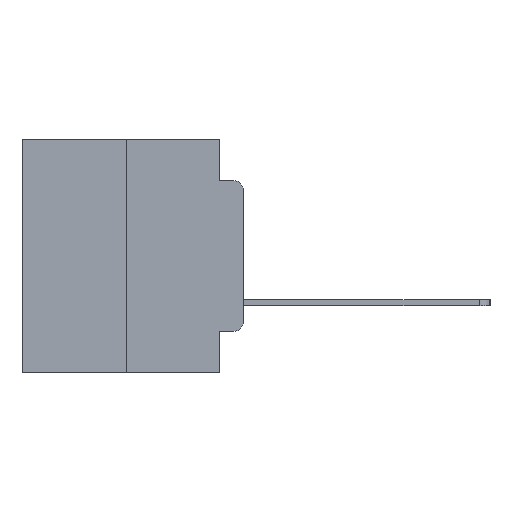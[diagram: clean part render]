
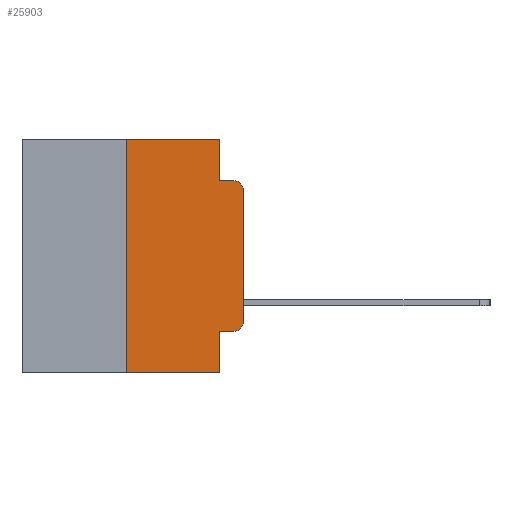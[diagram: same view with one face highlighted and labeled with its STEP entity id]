
A CAD part, left-side view. The second image highlights one B-rep face of the part: STEP entity #25903.
In plain terms, the highlighted planar face has unit normal (-1, 0, 0).
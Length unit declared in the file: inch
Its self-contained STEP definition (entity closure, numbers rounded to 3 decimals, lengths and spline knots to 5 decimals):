
#150 = CARTESIAN_POINT ( 'NONE',  ( 0., 0., -0.1085 ) ) ;
#372 = CARTESIAN_POINT ( 'NONE',  ( 0., 0.473, 0. ) ) ;
#815 = DIRECTION ( 'NONE',  ( 0., 0., 1. ) ) ;
#927 = DIRECTION ( 'NONE',  ( 0., 0., -1. ) ) ;
#1310 = CARTESIAN_POINT ( 'NONE',  ( 0., 0.02, -0.4115 ) ) ;
#1824 = CARTESIAN_POINT ( 'NONE',  ( 0., 0.02, -0.0885 ) ) ;
#1943 = CARTESIAN_POINT ( 'NONE',  ( 0., 0.051, 0. ) ) ;
#2210 = CIRCLE ( 'NONE', #12463, 0.02 ) ;
#2427 = CARTESIAN_POINT ( 'NONE',  ( 0., 0., 0. ) ) ;
#3663 = ORIENTED_EDGE ( 'NONE', *, *, #15110, .T. ) ;
#3817 = EDGE_CURVE ( 'NONE', #10203, #20519, #4267, .T. ) ;
#3851 = EDGE_CURVE ( 'NONE', #9845, #5851, #14530, .T. ) ;
#3986 = VECTOR ( 'NONE', #6783, 39.37008 ) ;
#4055 = DIRECTION ( 'NONE',  ( 0., 0., -1. ) ) ;
#4267 = CIRCLE ( 'NONE', #9182, 0.02 ) ;
#4334 = VECTOR ( 'NONE', #20975, 39.37008 ) ;
#4427 = CARTESIAN_POINT ( 'NONE',  ( 0., 0.051, 0. ) ) ;
#5043 = LINE ( 'NONE', #1943, #15949 ) ;
#5316 = CARTESIAN_POINT ( 'NONE',  ( 0., 0.25, -0.5 ) ) ;
#5504 = EDGE_CURVE ( 'NONE', #13456, #21660, #2210, .T. ) ;
#5851 = VERTEX_POINT ( 'NONE', #18523 ) ;
#6529 = CARTESIAN_POINT ( 'NONE',  ( 0., 0.051, -0.0885 ) ) ;
#6564 = EDGE_CURVE ( 'NONE', #21660, #10203, #19467, .T. ) ;
#6783 = DIRECTION ( 'NONE',  ( 0., -1., 0. ) ) ;
#7154 = VERTEX_POINT ( 'NONE', #18896 ) ;
#7891 = ORIENTED_EDGE ( 'NONE', *, *, #22722, .F. ) ;
#8489 = VECTOR ( 'NONE', #26136, 39.37008 ) ;
#8744 = ORIENTED_EDGE ( 'NONE', *, *, #20754, .F. ) ;
#9182 = AXIS2_PLACEMENT_3D ( 'NONE', #19022, #16588, #16552 ) ;
#9845 = VERTEX_POINT ( 'NONE', #5316 ) ;
#10203 = VERTEX_POINT ( 'NONE', #150 ) ;
#10524 = DIRECTION ( 'NONE',  ( 0., 0., -1. ) ) ;
#10583 = AXIS2_PLACEMENT_3D ( 'NONE', #372, #25048, #12928 ) ;
#11063 = LINE ( 'NONE', #11196, #17168 ) ;
#11196 = CARTESIAN_POINT ( 'NONE',  ( 0., 0.25, 0. ) ) ;
#12216 = ORIENTED_EDGE ( 'NONE', *, *, #3851, .T. ) ;
#12463 = AXIS2_PLACEMENT_3D ( 'NONE', #25460, #13337, #927 ) ;
#12928 = DIRECTION ( 'NONE',  ( 0., 0., -1. ) ) ;
#13304 = CARTESIAN_POINT ( 'NONE',  ( 0., 0.473, 0. ) ) ;
#13337 = DIRECTION ( 'NONE',  ( -1., 0., 0. ) ) ;
#13456 = VERTEX_POINT ( 'NONE', #1310 ) ;
#14033 = VECTOR ( 'NONE', #18833, 39.37008 ) ;
#14147 = ORIENTED_EDGE ( 'NONE', *, *, #26634, .F. ) ;
#14530 = LINE ( 'NONE', #24114, #8489 ) ;
#14685 = ORIENTED_EDGE ( 'NONE', *, *, #19396, .F. ) ;
#14887 = LINE ( 'NONE', #19015, #3986 ) ;
#15110 = EDGE_CURVE ( 'NONE', #23892, #13456, #14887, .T. ) ;
#15734 = CARTESIAN_POINT ( 'NONE',  ( 0., 0., -0.3915 ) ) ;
#15764 = VECTOR ( 'NONE', #25424, 39.37008 ) ;
#15949 = VECTOR ( 'NONE', #4055, 39.37008 ) ;
#16552 = DIRECTION ( 'NONE',  ( 0., 0., -1. ) ) ;
#16588 = DIRECTION ( 'NONE',  ( -1., 0., 0. ) ) ;
#16681 = ORIENTED_EDGE ( 'NONE', *, *, #25793, .F. ) ;
#17168 = VECTOR ( 'NONE', #815, 39.37008 ) ;
#17556 = VERTEX_POINT ( 'NONE', #4427 ) ;
#18173 = FACE_OUTER_BOUND ( 'NONE', #19398, .T. ) ;
#18523 = CARTESIAN_POINT ( 'NONE',  ( 0., 0.051, -0.5 ) ) ;
#18833 = DIRECTION ( 'NONE',  ( 0., 0., 1. ) ) ;
#18896 = CARTESIAN_POINT ( 'NONE',  ( 0., 0.25, 0. ) ) ;
#18992 = PLANE ( 'NONE',  #10583 ) ;
#19015 = CARTESIAN_POINT ( 'NONE',  ( 0., 0.051, -0.4115 ) ) ;
#19022 = CARTESIAN_POINT ( 'NONE',  ( 0., 0.02, -0.1085 ) ) ;
#19396 = EDGE_CURVE ( 'NONE', #17556, #25135, #5043, .T. ) ;
#19398 = EDGE_LOOP ( 'NONE', ( #24543, #20898, #8744, #14685, #7891, #14147, #12216, #16681, #3663, #24986 ) ) ;
#19406 = VECTOR ( 'NONE', #10524, 39.37008 ) ;
#19467 = LINE ( 'NONE', #2427, #14033 ) ;
#20519 = VERTEX_POINT ( 'NONE', #1824 ) ;
#20672 = CARTESIAN_POINT ( 'NONE',  ( 0., 0.051, 0. ) ) ;
#20754 = EDGE_CURVE ( 'NONE', #25135, #20519, #25324, .T. ) ;
#20898 = ORIENTED_EDGE ( 'NONE', *, *, #3817, .T. ) ;
#20975 = DIRECTION ( 'NONE',  ( 0., -1., 0. ) ) ;
#21660 = VERTEX_POINT ( 'NONE', #15734 ) ;
#22722 = EDGE_CURVE ( 'NONE', #7154, #17556, #25868, .T. ) ;
#23892 = VERTEX_POINT ( 'NONE', #24858 ) ;
#24114 = CARTESIAN_POINT ( 'NONE',  ( 0., 0.473, -0.5 ) ) ;
#24543 = ORIENTED_EDGE ( 'NONE', *, *, #6564, .T. ) ;
#24858 = CARTESIAN_POINT ( 'NONE',  ( 0., 0.051, -0.4115 ) ) ;
#24986 = ORIENTED_EDGE ( 'NONE', *, *, #5504, .T. ) ;
#25013 = CARTESIAN_POINT ( 'NONE',  ( 0., 0.051, -0.0885 ) ) ;
#25048 = DIRECTION ( 'NONE',  ( 1., 0., 0. ) ) ;
#25135 = VERTEX_POINT ( 'NONE', #6529 ) ;
#25324 = LINE ( 'NONE', #25013, #4334 ) ;
#25424 = DIRECTION ( 'NONE',  ( 0., -1., 0. ) ) ;
#25460 = CARTESIAN_POINT ( 'NONE',  ( 0., 0.02, -0.3915 ) ) ;
#25793 = EDGE_CURVE ( 'NONE', #23892, #5851, #26009, .T. ) ;
#25868 = LINE ( 'NONE', #13304, #15764 ) ;
#25903 = ADVANCED_FACE ( 'NONE', ( #18173 ), #18992, .F. ) ;
#26009 = LINE ( 'NONE', #20672, #19406 ) ;
#26136 = DIRECTION ( 'NONE',  ( 0., -1., 0. ) ) ;
#26634 = EDGE_CURVE ( 'NONE', #9845, #7154, #11063, .T. ) ;
